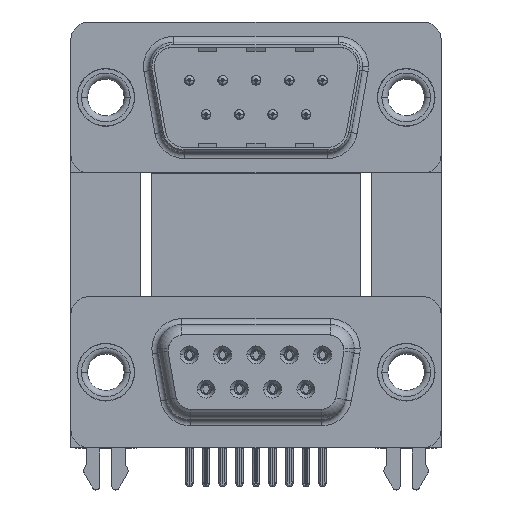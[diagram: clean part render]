
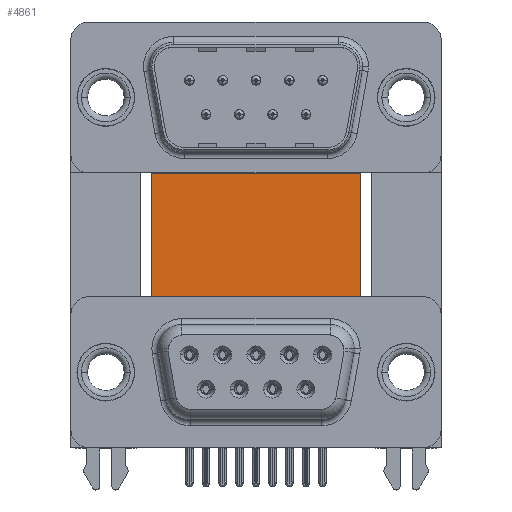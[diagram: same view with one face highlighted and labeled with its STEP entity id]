
A CAD part, top view. The second image highlights one B-rep face of the part: STEP entity #4861.
In plain terms, the highlighted planar face has unit normal (0, 0, 1).
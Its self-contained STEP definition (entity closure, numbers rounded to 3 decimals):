
#205 = CARTESIAN_POINT ( 'NONE',  ( 22.09, -4.635, -12. ) ) ;
#444 = VECTOR ( 'NONE', #30245, 1000. ) ;
#747 = CARTESIAN_POINT ( 'NONE',  ( 21.2, 16.585, -12. ) ) ;
#994 = CARTESIAN_POINT ( 'NONE',  ( 22.59, -4.635, -12. ) ) ;
#1577 = EDGE_CURVE ( 'NONE', #27421, #6498, #17174, .T. ) ;
#1853 = VERTEX_POINT ( 'NONE', #17660 ) ;
#2169 = ORIENTED_EDGE ( 'NONE', *, *, #22512, .T. ) ;
#3968 = VECTOR ( 'NONE', #7000, 1000. ) ;
#4861 = ADVANCED_FACE ( 'NONE', ( #19831 ), #5564, .F. ) ;
#5161 = LINE ( 'NONE', #36318, #27871 ) ;
#5542 = VERTEX_POINT ( 'NONE', #205 ) ;
#5564 = PLANE ( 'NONE',  #19924 ) ;
#6211 = DIRECTION ( 'NONE',  ( -0.336, -0.942, 0. ) ) ;
#6246 = EDGE_CURVE ( 'NONE', #1853, #27421, #18133, .T. ) ;
#6333 = DIRECTION ( 'NONE',  ( 0., -1., 0. ) ) ;
#6385 = CARTESIAN_POINT ( 'NONE',  ( 2.4, -4.635, -12. ) ) ;
#6498 = VERTEX_POINT ( 'NONE', #30316 ) ;
#7000 = DIRECTION ( 'NONE',  ( 0., -1., 0. ) ) ;
#7002 = CARTESIAN_POINT ( 'NONE',  ( 21.2, 16.585, -12. ) ) ;
#7030 = DIRECTION ( 'NONE',  ( 0., 1., 0. ) ) ;
#7744 = VECTOR ( 'NONE', #23106, 1000. ) ;
#7758 = DIRECTION ( 'NONE',  ( 1., 0., 0. ) ) ;
#7977 = DIRECTION ( 'NONE',  ( 0., 0., -1. ) ) ;
#8317 = ORIENTED_EDGE ( 'NONE', *, *, #8468, .T. ) ;
#8468 = EDGE_CURVE ( 'NONE', #24848, #32099, #23914, .T. ) ;
#9716 = ORIENTED_EDGE ( 'NONE', *, *, #1577, .T. ) ;
#9778 = VECTOR ( 'NONE', #12880, 1000. ) ;
#10076 = VERTEX_POINT ( 'NONE', #16476 ) ;
#10383 = CARTESIAN_POINT ( 'NONE',  ( 2.9, -3.735, -12. ) ) ;
#11136 = DIRECTION ( 'NONE',  ( -1., 0., 0. ) ) ;
#12035 = VERTEX_POINT ( 'NONE', #15087 ) ;
#12516 = EDGE_LOOP ( 'NONE', ( #8317, #2169, #29929, #21252, #33663, #12553, #19282, #9716, #21556, #34523 ) ) ;
#12553 = ORIENTED_EDGE ( 'NONE', *, *, #35013, .F. ) ;
#12843 = VECTOR ( 'NONE', #7030, 1000. ) ;
#12880 = DIRECTION ( 'NONE',  ( 1., 0., 0. ) ) ;
#12988 = LINE ( 'NONE', #10383, #12843 ) ;
#13328 = EDGE_CURVE ( 'NONE', #6498, #12035, #21570, .T. ) ;
#13440 = CARTESIAN_POINT ( 'NONE',  ( 2.9, -4.635, -12. ) ) ;
#13768 = LINE ( 'NONE', #16180, #23811 ) ;
#15087 = CARTESIAN_POINT ( 'NONE',  ( 2.9, -4.635, -12. ) ) ;
#16180 = CARTESIAN_POINT ( 'NONE',  ( 22.09, -4.635, -12. ) ) ;
#16476 = CARTESIAN_POINT ( 'NONE',  ( 21.2, -0.735, -12. ) ) ;
#16876 = CARTESIAN_POINT ( 'NONE',  ( 3.79, 16.585, -12. ) ) ;
#17153 = EDGE_CURVE ( 'NONE', #5542, #35710, #13768, .T. ) ;
#17174 = LINE ( 'NONE', #6385, #21440 ) ;
#17660 = CARTESIAN_POINT ( 'NONE',  ( 3.79, 16.585, -12. ) ) ;
#18133 = LINE ( 'NONE', #32796, #3968 ) ;
#19282 = ORIENTED_EDGE ( 'NONE', *, *, #6246, .T. ) ;
#19831 = FACE_OUTER_BOUND ( 'NONE', #12516, .T. ) ;
#19924 = AXIS2_PLACEMENT_3D ( 'NONE', #16876, #7977, #11136 ) ;
#21135 = CARTESIAN_POINT ( 'NONE',  ( 22.09, -3.735, -12. ) ) ;
#21252 = ORIENTED_EDGE ( 'NONE', *, *, #27342, .T. ) ;
#21304 = CARTESIAN_POINT ( 'NONE',  ( 3.79, -3.735, -12. ) ) ;
#21440 = VECTOR ( 'NONE', #6211, 1000. ) ;
#21556 = ORIENTED_EDGE ( 'NONE', *, *, #13328, .T. ) ;
#21570 = LINE ( 'NONE', #13440, #9778 ) ;
#22281 = EDGE_CURVE ( 'NONE', #34779, #10076, #23035, .T. ) ;
#22494 = VECTOR ( 'NONE', #30045, 1000. ) ;
#22512 = EDGE_CURVE ( 'NONE', #32099, #5542, #23924, .T. ) ;
#23035 = LINE ( 'NONE', #747, #36003 ) ;
#23106 = DIRECTION ( 'NONE',  ( -0.336, 0.942, 0. ) ) ;
#23811 = VECTOR ( 'NONE', #27475, 1000. ) ;
#23914 = LINE ( 'NONE', #21304, #22494 ) ;
#23924 = LINE ( 'NONE', #21135, #444 ) ;
#24305 = CARTESIAN_POINT ( 'NONE',  ( 2.9, -3.735, -12. ) ) ;
#24848 = VERTEX_POINT ( 'NONE', #24305 ) ;
#26238 = LINE ( 'NONE', #994, #7744 ) ;
#27342 = EDGE_CURVE ( 'NONE', #35710, #10076, #26238, .T. ) ;
#27421 = VERTEX_POINT ( 'NONE', #28849 ) ;
#27475 = DIRECTION ( 'NONE',  ( 1., 0., 0. ) ) ;
#27871 = VECTOR ( 'NONE', #7758, 1000. ) ;
#28849 = CARTESIAN_POINT ( 'NONE',  ( 3.79, -0.735, -12. ) ) ;
#28891 = CARTESIAN_POINT ( 'NONE',  ( 22.09, -3.735, -12. ) ) ;
#29363 = CARTESIAN_POINT ( 'NONE',  ( 22.59, -4.635, -12. ) ) ;
#29929 = ORIENTED_EDGE ( 'NONE', *, *, #17153, .T. ) ;
#30045 = DIRECTION ( 'NONE',  ( 1., 0., 0. ) ) ;
#30245 = DIRECTION ( 'NONE',  ( 0., -1., 0. ) ) ;
#30316 = CARTESIAN_POINT ( 'NONE',  ( 2.4, -4.635, -12. ) ) ;
#31840 = EDGE_CURVE ( 'NONE', #12035, #24848, #12988, .T. ) ;
#32099 = VERTEX_POINT ( 'NONE', #28891 ) ;
#32796 = CARTESIAN_POINT ( 'NONE',  ( 3.79, 16.585, -12. ) ) ;
#33663 = ORIENTED_EDGE ( 'NONE', *, *, #22281, .F. ) ;
#34523 = ORIENTED_EDGE ( 'NONE', *, *, #31840, .T. ) ;
#34779 = VERTEX_POINT ( 'NONE', #7002 ) ;
#35013 = EDGE_CURVE ( 'NONE', #1853, #34779, #5161, .T. ) ;
#35710 = VERTEX_POINT ( 'NONE', #29363 ) ;
#36003 = VECTOR ( 'NONE', #6333, 1000. ) ;
#36318 = CARTESIAN_POINT ( 'NONE',  ( 3.79, 16.585, -12. ) ) ;
